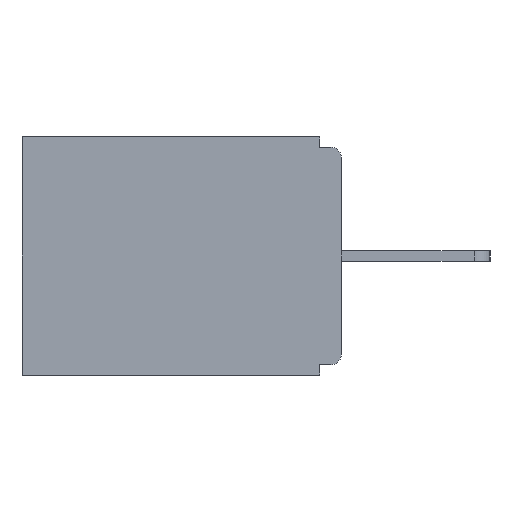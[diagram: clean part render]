
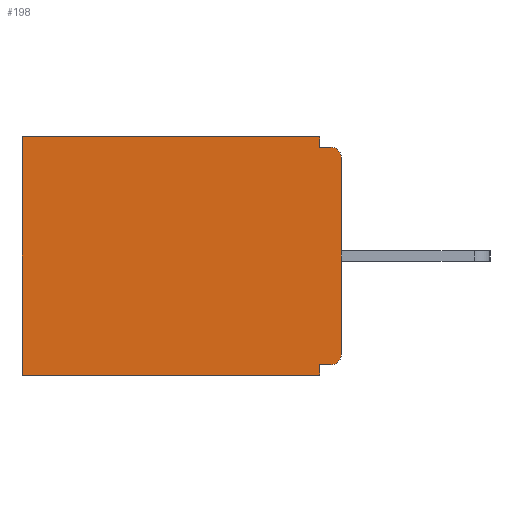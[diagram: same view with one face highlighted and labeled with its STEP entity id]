
A CAD part, left-side view. The second image highlights one B-rep face of the part: STEP entity #198.
In plain terms, the highlighted planar face has unit normal (-1, 0, 0).
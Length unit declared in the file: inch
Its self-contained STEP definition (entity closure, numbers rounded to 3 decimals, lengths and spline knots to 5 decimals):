
#60 = LINE ( 'NONE', #5493, #2091 ) ;
#131 = VERTEX_POINT ( 'NONE', #6345 ) ;
#198 = ADVANCED_FACE ( 'NONE', ( #393 ), #10044, .F. ) ;
#393 = FACE_OUTER_BOUND ( 'NONE', #1966, .T. ) ;
#422 = VERTEX_POINT ( 'NONE', #6808 ) ;
#1093 = ORIENTED_EDGE ( 'NONE', *, *, #10961, .F. ) ;
#1131 = AXIS2_PLACEMENT_3D ( 'NONE', #6578, #4700, #7521 ) ;
#1245 = LINE ( 'NONE', #4033, #10507 ) ;
#1321 = CARTESIAN_POINT ( 'NONE',  ( 0.298, 0.015, -0.015 ) ) ;
#1364 = DIRECTION ( 'NONE',  ( 0., 0., -1. ) ) ;
#1401 = CARTESIAN_POINT ( 'NONE',  ( 0.298, 0.015, -0.328 ) ) ;
#1614 = DIRECTION ( 'NONE',  ( 0., 0., -1. ) ) ;
#1783 = CARTESIAN_POINT ( 'NONE',  ( 0.298, 0.031, -0.343 ) ) ;
#1824 = LINE ( 'NONE', #5383, #7905 ) ;
#1966 = EDGE_LOOP ( 'NONE', ( #2343, #2088, #10786, #2646, #6218, #10541, #10279, #7581, #6110, #1093 ) ) ;
#2049 = VERTEX_POINT ( 'NONE', #10410 ) ;
#2088 = ORIENTED_EDGE ( 'NONE', *, *, #8484, .F. ) ;
#2091 = VECTOR ( 'NONE', #2688, 39.37008 ) ;
#2343 = ORIENTED_EDGE ( 'NONE', *, *, #4818, .T. ) ;
#2529 = VERTEX_POINT ( 'NONE', #7830 ) ;
#2646 = ORIENTED_EDGE ( 'NONE', *, *, #6825, .T. ) ;
#2688 = DIRECTION ( 'NONE',  ( 0., 0., -1. ) ) ;
#2737 = CIRCLE ( 'NONE', #11321, 0.015 ) ;
#2802 = CARTESIAN_POINT ( 'NONE',  ( 0.298, 0., 0. ) ) ;
#2922 = DIRECTION ( 'NONE',  ( -1., 0., 0. ) ) ;
#3023 = CARTESIAN_POINT ( 'NONE',  ( 0.298, 0., -0.015 ) ) ;
#3883 = LINE ( 'NONE', #3023, #10695 ) ;
#3956 = CARTESIAN_POINT ( 'NONE',  ( 0.298, 0.015, -0.313 ) ) ;
#3990 = VECTOR ( 'NONE', #7992, 39.37008 ) ;
#4033 = CARTESIAN_POINT ( 'NONE',  ( 0.298, 0., 0. ) ) ;
#4539 = EDGE_CURVE ( 'NONE', #8436, #9814, #8275, .T. ) ;
#4700 = DIRECTION ( 'NONE',  ( 1., 0., 0. ) ) ;
#4796 = CARTESIAN_POINT ( 'NONE',  ( 0.298, 0., -0.03 ) ) ;
#4818 = EDGE_CURVE ( 'NONE', #9522, #7826, #2737, .T. ) ;
#4890 = EDGE_CURVE ( 'NONE', #422, #2049, #8692, .T. ) ;
#5375 = DIRECTION ( 'NONE',  ( 0., 0., -1. ) ) ;
#5383 = CARTESIAN_POINT ( 'NONE',  ( 0.298, 0., -0.343 ) ) ;
#5493 = CARTESIAN_POINT ( 'NONE',  ( 0.298, 0.031, -0.343 ) ) ;
#6110 = ORIENTED_EDGE ( 'NONE', *, *, #9940, .T. ) ;
#6205 = DIRECTION ( 'NONE',  ( 0., 1., 0. ) ) ;
#6218 = ORIENTED_EDGE ( 'NONE', *, *, #4539, .T. ) ;
#6345 = CARTESIAN_POINT ( 'NONE',  ( 0.298, 0., -0.313 ) ) ;
#6481 = DIRECTION ( 'NONE',  ( 0., -1., 0. ) ) ;
#6578 = CARTESIAN_POINT ( 'NONE',  ( 0.298, 0., 0. ) ) ;
#6658 = DIRECTION ( 'NONE',  ( 0., 0., -1. ) ) ;
#6709 = EDGE_CURVE ( 'NONE', #2529, #9814, #1824, .T. ) ;
#6726 = DIRECTION ( 'NONE',  ( 0., 1., 0. ) ) ;
#6808 = CARTESIAN_POINT ( 'NONE',  ( 0.298, 0.031, 0. ) ) ;
#6825 = EDGE_CURVE ( 'NONE', #422, #8436, #1245, .T. ) ;
#7185 = LINE ( 'NONE', #2802, #10097 ) ;
#7521 = DIRECTION ( 'NONE',  ( 0., 0., -1. ) ) ;
#7581 = ORIENTED_EDGE ( 'NONE', *, *, #9723, .F. ) ;
#7616 = LINE ( 'NONE', #11174, #11083 ) ;
#7826 = VERTEX_POINT ( 'NONE', #1321 ) ;
#7830 = CARTESIAN_POINT ( 'NONE',  ( 0.298, 0.031, -0.343 ) ) ;
#7905 = VECTOR ( 'NONE', #6205, 39.37008 ) ;
#7944 = CIRCLE ( 'NONE', #9060, 0.015 ) ;
#7992 = DIRECTION ( 'NONE',  ( 0., 0., -1. ) ) ;
#8253 = VERTEX_POINT ( 'NONE', #10204 ) ;
#8275 = LINE ( 'NONE', #8335, #10488 ) ;
#8335 = CARTESIAN_POINT ( 'NONE',  ( 0.298, 0.46, 0. ) ) ;
#8400 = EDGE_CURVE ( 'NONE', #8253, #2529, #60, .T. ) ;
#8436 = VERTEX_POINT ( 'NONE', #9885 ) ;
#8484 = EDGE_CURVE ( 'NONE', #2049, #7826, #3883, .T. ) ;
#8503 = DIRECTION ( 'NONE',  ( 0., 1., 0. ) ) ;
#8692 = LINE ( 'NONE', #1783, #3990 ) ;
#9060 = AXIS2_PLACEMENT_3D ( 'NONE', #3956, #2922, #6658 ) ;
#9522 = VERTEX_POINT ( 'NONE', #4796 ) ;
#9682 = DIRECTION ( 'NONE',  ( -1., 0., 0. ) ) ;
#9723 = EDGE_CURVE ( 'NONE', #10110, #8253, #7616, .T. ) ;
#9814 = VERTEX_POINT ( 'NONE', #10599 ) ;
#9885 = CARTESIAN_POINT ( 'NONE',  ( 0.298, 0.46, 0. ) ) ;
#9940 = EDGE_CURVE ( 'NONE', #10110, #131, #7944, .T. ) ;
#10044 = PLANE ( 'NONE',  #1131 ) ;
#10097 = VECTOR ( 'NONE', #5375, 39.37008 ) ;
#10110 = VERTEX_POINT ( 'NONE', #1401 ) ;
#10204 = CARTESIAN_POINT ( 'NONE',  ( 0.298, 0.031, -0.328 ) ) ;
#10279 = ORIENTED_EDGE ( 'NONE', *, *, #8400, .F. ) ;
#10410 = CARTESIAN_POINT ( 'NONE',  ( 0.298, 0.031, -0.015 ) ) ;
#10488 = VECTOR ( 'NONE', #1364, 39.37008 ) ;
#10507 = VECTOR ( 'NONE', #8503, 39.37008 ) ;
#10541 = ORIENTED_EDGE ( 'NONE', *, *, #6709, .F. ) ;
#10599 = CARTESIAN_POINT ( 'NONE',  ( 0.298, 0.46, -0.343 ) ) ;
#10695 = VECTOR ( 'NONE', #6481, 39.37008 ) ;
#10786 = ORIENTED_EDGE ( 'NONE', *, *, #4890, .F. ) ;
#10961 = EDGE_CURVE ( 'NONE', #9522, #131, #7185, .T. ) ;
#11083 = VECTOR ( 'NONE', #6726, 39.37008 ) ;
#11174 = CARTESIAN_POINT ( 'NONE',  ( 0.298, 0., -0.328 ) ) ;
#11321 = AXIS2_PLACEMENT_3D ( 'NONE', #11484, #9682, #1614 ) ;
#11484 = CARTESIAN_POINT ( 'NONE',  ( 0.298, 0.015, -0.03 ) ) ;
